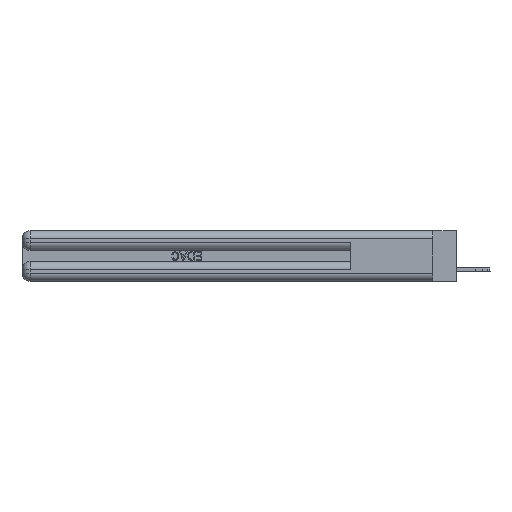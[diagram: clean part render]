
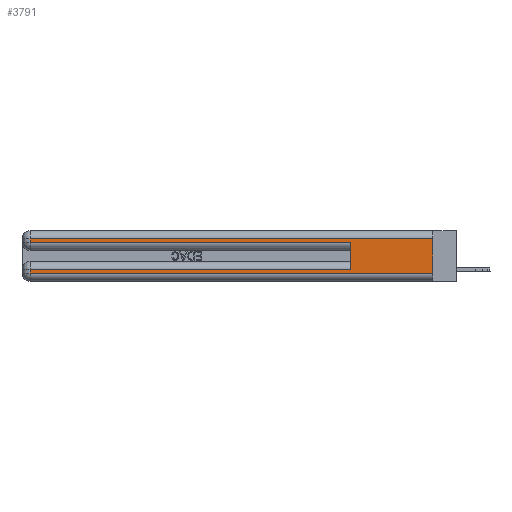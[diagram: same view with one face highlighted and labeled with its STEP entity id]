
A CAD part, left-side view. The second image highlights one B-rep face of the part: STEP entity #3791.
In plain terms, the highlighted planar face has unit normal (-1, 0, 0).
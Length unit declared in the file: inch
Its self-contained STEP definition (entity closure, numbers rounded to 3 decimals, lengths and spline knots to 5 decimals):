
#323 = CARTESIAN_POINT ( 'NONE',  ( 0., 0., 0.285 ) ) ;
#399 = VECTOR ( 'NONE', #27105, 39.37008 ) ;
#1755 = CARTESIAN_POINT ( 'NONE',  ( 0., 0., 0.31 ) ) ;
#2781 = EDGE_CURVE ( 'NONE', #2864, #26411, #6257, .T. ) ;
#2864 = VERTEX_POINT ( 'NONE', #14405 ) ;
#3053 = ORIENTED_EDGE ( 'NONE', *, *, #23860, .F. ) ;
#3791 = ADVANCED_FACE ( 'NONE', ( #4438 ), #19758, .F. ) ;
#4024 = VERTEX_POINT ( 'NONE', #25251 ) ;
#4438 = FACE_OUTER_BOUND ( 'NONE', #17873, .T. ) ;
#4716 = DIRECTION ( 'NONE',  ( 0., 0., -1. ) ) ;
#5733 = AXIS2_PLACEMENT_3D ( 'NONE', #14923, #18384, #24600 ) ;
#6063 = VECTOR ( 'NONE', #4716, 39.37008 ) ;
#6257 = LINE ( 'NONE', #33008, #27640 ) ;
#6382 = CARTESIAN_POINT ( 'NONE',  ( 0., 2.94, 0.37 ) ) ;
#7299 = CARTESIAN_POINT ( 'NONE',  ( 0., 0., 0.37 ) ) ;
#7650 = EDGE_CURVE ( 'NONE', #20995, #17010, #33383, .T. ) ;
#7851 = CARTESIAN_POINT ( 'NONE',  ( 0., 2.94, 0.37 ) ) ;
#7966 = VECTOR ( 'NONE', #23253, 39.37008 ) ;
#8026 = ORIENTED_EDGE ( 'NONE', *, *, #7650, .T. ) ;
#9354 = ORIENTED_EDGE ( 'NONE', *, *, #13443, .T. ) ;
#9669 = DIRECTION ( 'NONE',  ( 0., 1., 0. ) ) ;
#10552 = LINE ( 'NONE', #7851, #32380 ) ;
#11681 = DIRECTION ( 'NONE',  ( 0., -1., 0. ) ) ;
#11705 = ORIENTED_EDGE ( 'NONE', *, *, #28661, .T. ) ;
#12562 = ORIENTED_EDGE ( 'NONE', *, *, #2781, .T. ) ;
#12974 = CARTESIAN_POINT ( 'NONE',  ( 0., 2.94, 0.285 ) ) ;
#13443 = EDGE_CURVE ( 'NONE', #19689, #4024, #18564, .T. ) ;
#14405 = CARTESIAN_POINT ( 'NONE',  ( 0., 0.6, 0.085 ) ) ;
#14794 = EDGE_CURVE ( 'NONE', #26411, #19689, #10552, .T. ) ;
#14923 = CARTESIAN_POINT ( 'NONE',  ( 0., 0., 0.37 ) ) ;
#15242 = CARTESIAN_POINT ( 'NONE',  ( 0., 0.6, 0.145 ) ) ;
#16122 = VERTEX_POINT ( 'NONE', #1755 ) ;
#16580 = CARTESIAN_POINT ( 'NONE',  ( 0., 0.6, 0.285 ) ) ;
#17010 = VERTEX_POINT ( 'NONE', #12974 ) ;
#17873 = EDGE_LOOP ( 'NONE', ( #21060, #30974, #8026, #11705, #3053, #12562, #33479, #9354 ) ) ;
#17917 = CARTESIAN_POINT ( 'NONE',  ( 0., 2.94, 0.085 ) ) ;
#18384 = DIRECTION ( 'NONE',  ( 1., 0., 0. ) ) ;
#18470 = CARTESIAN_POINT ( 'NONE',  ( 0., 0., 0.31 ) ) ;
#18564 = LINE ( 'NONE', #23276, #399 ) ;
#19689 = VERTEX_POINT ( 'NONE', #33992 ) ;
#19758 = PLANE ( 'NONE',  #5733 ) ;
#20376 = CARTESIAN_POINT ( 'NONE',  ( 0., 2.94, 0.31 ) ) ;
#20665 = EDGE_CURVE ( 'NONE', #16122, #4024, #24725, .T. ) ;
#20969 = DIRECTION ( 'NONE',  ( 0., 0., 1. ) ) ;
#20995 = VERTEX_POINT ( 'NONE', #20376 ) ;
#21060 = ORIENTED_EDGE ( 'NONE', *, *, #20665, .F. ) ;
#23253 = DIRECTION ( 'NONE',  ( 0., 0., -1. ) ) ;
#23276 = CARTESIAN_POINT ( 'NONE',  ( 0., 0., 0.06 ) ) ;
#23812 = EDGE_CURVE ( 'NONE', #16122, #20995, #32571, .T. ) ;
#23860 = EDGE_CURVE ( 'NONE', #2864, #32327, #25401, .T. ) ;
#24600 = DIRECTION ( 'NONE',  ( 0., 0., -1. ) ) ;
#24725 = LINE ( 'NONE', #7299, #6063 ) ;
#25251 = CARTESIAN_POINT ( 'NONE',  ( 0., 0., 0.06 ) ) ;
#25354 = VECTOR ( 'NONE', #11681, 39.37008 ) ;
#25401 = LINE ( 'NONE', #15242, #31678 ) ;
#25875 = VECTOR ( 'NONE', #9669, 39.37008 ) ;
#26411 = VERTEX_POINT ( 'NONE', #17917 ) ;
#27105 = DIRECTION ( 'NONE',  ( 0., -1., 0. ) ) ;
#27640 = VECTOR ( 'NONE', #30154, 39.37008 ) ;
#28661 = EDGE_CURVE ( 'NONE', #17010, #32327, #32949, .T. ) ;
#30154 = DIRECTION ( 'NONE',  ( 0., 1., 0. ) ) ;
#30760 = DIRECTION ( 'NONE',  ( 0., 0., -1. ) ) ;
#30974 = ORIENTED_EDGE ( 'NONE', *, *, #23812, .T. ) ;
#31678 = VECTOR ( 'NONE', #20969, 39.37008 ) ;
#32327 = VERTEX_POINT ( 'NONE', #16580 ) ;
#32380 = VECTOR ( 'NONE', #30760, 39.37008 ) ;
#32571 = LINE ( 'NONE', #18470, #25875 ) ;
#32949 = LINE ( 'NONE', #323, #25354 ) ;
#33008 = CARTESIAN_POINT ( 'NONE',  ( 0., 0., 0.085 ) ) ;
#33383 = LINE ( 'NONE', #6382, #7966 ) ;
#33479 = ORIENTED_EDGE ( 'NONE', *, *, #14794, .T. ) ;
#33992 = CARTESIAN_POINT ( 'NONE',  ( 0., 2.94, 0.06 ) ) ;
